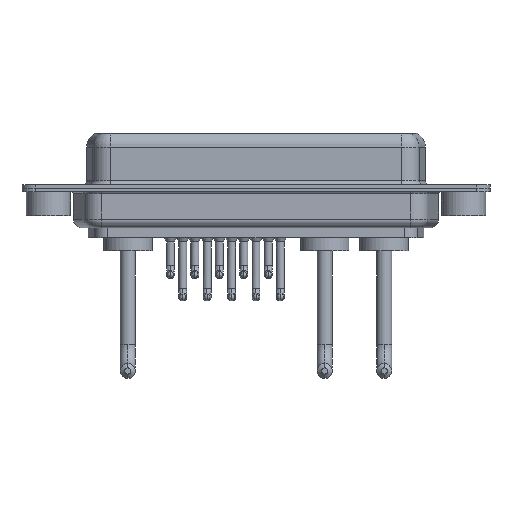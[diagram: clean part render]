
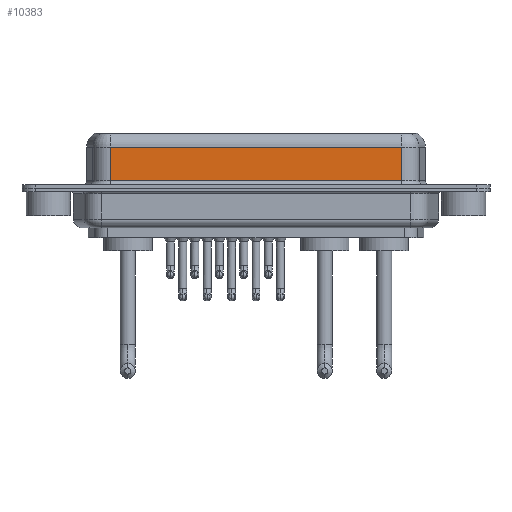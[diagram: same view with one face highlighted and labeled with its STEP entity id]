
A CAD part, front view. The second image highlights one B-rep face of the part: STEP entity #10383.
In plain terms, the highlighted planar face has unit normal (0, -1, 0).
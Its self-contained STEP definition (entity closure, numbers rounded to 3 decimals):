
#301 = VERTEX_POINT ( 'NONE', #780 ) ;
#780 = CARTESIAN_POINT ( 'NONE',  ( 40.037, -3.95, 4.65 ) ) ;
#1268 = DIRECTION ( 'NONE',  ( -1., 0., 0. ) ) ;
#1997 = CARTESIAN_POINT ( 'NONE',  ( 40.037, -3.95, 0.9 ) ) ;
#2812 = FACE_OUTER_BOUND ( 'NONE', #11428, .T. ) ;
#4174 = LINE ( 'NONE', #15739, #5678 ) ;
#4338 = LINE ( 'NONE', #14646, #9864 ) ;
#4536 = DIRECTION ( 'NONE',  ( 0., 1., 0. ) ) ;
#4960 = EDGE_CURVE ( 'NONE', #301, #6731, #4174, .T. ) ;
#5069 = AXIS2_PLACEMENT_3D ( 'NONE', #17728, #4536, #5580 ) ;
#5580 = DIRECTION ( 'NONE',  ( 0., 0., 1. ) ) ;
#5678 = VECTOR ( 'NONE', #1268, 1000. ) ;
#5720 = EDGE_CURVE ( 'NONE', #6731, #15210, #6188, .T. ) ;
#6188 = LINE ( 'NONE', #15357, #13480 ) ;
#6731 = VERTEX_POINT ( 'NONE', #8412 ) ;
#7642 = ORIENTED_EDGE ( 'NONE', *, *, #16049, .F. ) ;
#7908 = ORIENTED_EDGE ( 'NONE', *, *, #18859, .T. ) ;
#8412 = CARTESIAN_POINT ( 'NONE',  ( 7.013, -3.95, 4.65 ) ) ;
#9011 = CARTESIAN_POINT ( 'NONE',  ( 40.037, -3.95, 6.4 ) ) ;
#9864 = VECTOR ( 'NONE', #16098, 1000. ) ;
#10383 = ADVANCED_FACE ( 'NONE', ( #2812 ), #18799, .F. ) ;
#10442 = ORIENTED_EDGE ( 'NONE', *, *, #4960, .T. ) ;
#10731 = VERTEX_POINT ( 'NONE', #1997 ) ;
#11428 = EDGE_LOOP ( 'NONE', ( #7642, #10442, #18771, #7908 ) ) ;
#11661 = LINE ( 'NONE', #9011, #13825 ) ;
#12182 = CARTESIAN_POINT ( 'NONE',  ( 7.013, -3.95, 0.9 ) ) ;
#12189 = DIRECTION ( 'NONE',  ( 0., 0., -1. ) ) ;
#13480 = VECTOR ( 'NONE', #12189, 1000. ) ;
#13825 = VECTOR ( 'NONE', #18955, 1000. ) ;
#14646 = CARTESIAN_POINT ( 'NONE',  ( 40.037, -3.95, 0.9 ) ) ;
#15210 = VERTEX_POINT ( 'NONE', #12182 ) ;
#15357 = CARTESIAN_POINT ( 'NONE',  ( 7.013, -3.95, 6.4 ) ) ;
#15739 = CARTESIAN_POINT ( 'NONE',  ( 40.037, -3.95, 4.65 ) ) ;
#16049 = EDGE_CURVE ( 'NONE', #301, #10731, #11661, .T. ) ;
#16098 = DIRECTION ( 'NONE',  ( 1., 0., 0. ) ) ;
#17728 = CARTESIAN_POINT ( 'NONE',  ( 40.037, -3.95, 6.4 ) ) ;
#18771 = ORIENTED_EDGE ( 'NONE', *, *, #5720, .T. ) ;
#18799 = PLANE ( 'NONE',  #5069 ) ;
#18859 = EDGE_CURVE ( 'NONE', #15210, #10731, #4338, .T. ) ;
#18955 = DIRECTION ( 'NONE',  ( 0., 0., -1. ) ) ;
